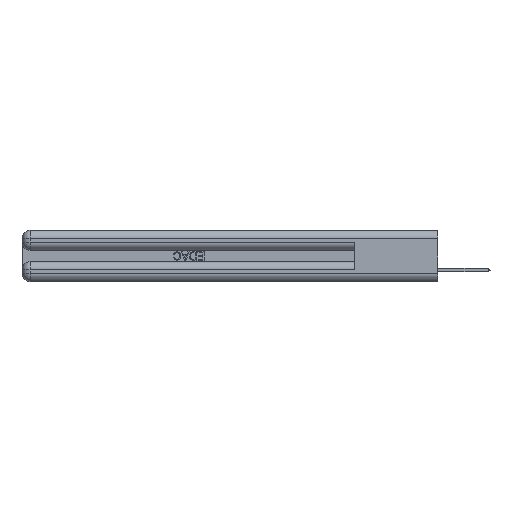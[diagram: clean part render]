
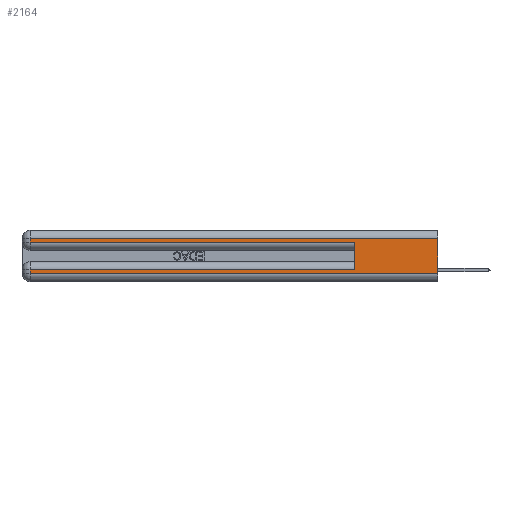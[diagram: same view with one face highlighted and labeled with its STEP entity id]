
A CAD part, left-side view. The second image highlights one B-rep face of the part: STEP entity #2164.
In plain terms, the highlighted planar face has unit normal (-1, 0, 0).
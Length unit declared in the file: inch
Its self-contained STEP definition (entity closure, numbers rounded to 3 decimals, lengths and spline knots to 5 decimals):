
#159 = EDGE_CURVE ( 'NONE', #7602, #18989, #10091, .T. ) ;
#1267 = LINE ( 'NONE', #23984, #44156 ) ;
#2164 = ADVANCED_FACE ( 'NONE', ( #12031 ), #34060, .F. ) ;
#2642 = ORIENTED_EDGE ( 'NONE', *, *, #159, .T. ) ;
#2807 = ORIENTED_EDGE ( 'NONE', *, *, #13919, .F. ) ;
#2818 = EDGE_CURVE ( 'NONE', #22507, #7602, #30417, .T. ) ;
#3405 = ORIENTED_EDGE ( 'NONE', *, *, #26136, .T. ) ;
#4474 = CARTESIAN_POINT ( 'NONE',  ( 0., 0.6, 0.145 ) ) ;
#4896 = AXIS2_PLACEMENT_3D ( 'NONE', #23490, #34382, #41384 ) ;
#6411 = EDGE_CURVE ( 'NONE', #44815, #10000, #44076, .T. ) ;
#6507 = CARTESIAN_POINT ( 'NONE',  ( 0., 0., 0.37 ) ) ;
#6776 = DIRECTION ( 'NONE',  ( 0., 1., 0. ) ) ;
#7141 = CARTESIAN_POINT ( 'NONE',  ( 0., 0.6, 0.085 ) ) ;
#7232 = CARTESIAN_POINT ( 'NONE',  ( 0., 0., 0.06 ) ) ;
#7307 = LINE ( 'NONE', #16290, #10110 ) ;
#7602 = VERTEX_POINT ( 'NONE', #23586 ) ;
#8119 = EDGE_CURVE ( 'NONE', #18989, #27806, #22187, .T. ) ;
#9535 = ORIENTED_EDGE ( 'NONE', *, *, #2818, .T. ) ;
#10000 = VERTEX_POINT ( 'NONE', #22575 ) ;
#10091 = LINE ( 'NONE', #32590, #18378 ) ;
#10110 = VECTOR ( 'NONE', #44787, 39.37008 ) ;
#10791 = DIRECTION ( 'NONE',  ( 0., 0., -1. ) ) ;
#12031 = FACE_OUTER_BOUND ( 'NONE', #30155, .T. ) ;
#12616 = CARTESIAN_POINT ( 'NONE',  ( 0., 0.6, 0.285 ) ) ;
#12782 = VECTOR ( 'NONE', #21292, 39.37008 ) ;
#13919 = EDGE_CURVE ( 'NONE', #22507, #20232, #15907, .T. ) ;
#15163 = CARTESIAN_POINT ( 'NONE',  ( 0., 2.94, 0.06 ) ) ;
#15520 = EDGE_CURVE ( 'NONE', #10000, #19739, #1267, .T. ) ;
#15907 = LINE ( 'NONE', #6507, #18165 ) ;
#16290 = CARTESIAN_POINT ( 'NONE',  ( 0., 0., 0.06 ) ) ;
#16591 = ORIENTED_EDGE ( 'NONE', *, *, #15520, .T. ) ;
#17574 = DIRECTION ( 'NONE',  ( 0., 1., 0. ) ) ;
#18165 = VECTOR ( 'NONE', #10791, 39.37008 ) ;
#18378 = VECTOR ( 'NONE', #40500, 39.37008 ) ;
#18989 = VERTEX_POINT ( 'NONE', #19274 ) ;
#19274 = CARTESIAN_POINT ( 'NONE',  ( 0., 2.94, 0.285 ) ) ;
#19739 = VERTEX_POINT ( 'NONE', #15163 ) ;
#20232 = VERTEX_POINT ( 'NONE', #7232 ) ;
#20900 = EDGE_CURVE ( 'NONE', #44815, #27806, #31871, .T. ) ;
#21292 = DIRECTION ( 'NONE',  ( 0., -1., 0. ) ) ;
#21804 = VECTOR ( 'NONE', #6776, 39.37008 ) ;
#22187 = LINE ( 'NONE', #44348, #12782 ) ;
#22360 = VECTOR ( 'NONE', #33080, 39.37008 ) ;
#22507 = VERTEX_POINT ( 'NONE', #27233 ) ;
#22575 = CARTESIAN_POINT ( 'NONE',  ( 0., 2.94, 0.085 ) ) ;
#23191 = VECTOR ( 'NONE', #17574, 39.37008 ) ;
#23490 = CARTESIAN_POINT ( 'NONE',  ( 0., 0., 0.37 ) ) ;
#23586 = CARTESIAN_POINT ( 'NONE',  ( 0., 2.94, 0.31 ) ) ;
#23871 = ORIENTED_EDGE ( 'NONE', *, *, #6411, .T. ) ;
#23984 = CARTESIAN_POINT ( 'NONE',  ( 0., 2.94, 0.37 ) ) ;
#24438 = CARTESIAN_POINT ( 'NONE',  ( 0., 0., 0.31 ) ) ;
#24493 = ORIENTED_EDGE ( 'NONE', *, *, #20900, .F. ) ;
#26136 = EDGE_CURVE ( 'NONE', #19739, #20232, #7307, .T. ) ;
#27233 = CARTESIAN_POINT ( 'NONE',  ( 0., 0., 0.31 ) ) ;
#27806 = VERTEX_POINT ( 'NONE', #12616 ) ;
#28037 = CARTESIAN_POINT ( 'NONE',  ( 0., 0., 0.085 ) ) ;
#30155 = EDGE_LOOP ( 'NONE', ( #2807, #9535, #2642, #40774, #24493, #23871, #16591, #3405 ) ) ;
#30417 = LINE ( 'NONE', #24438, #23191 ) ;
#31871 = LINE ( 'NONE', #4474, #22360 ) ;
#32590 = CARTESIAN_POINT ( 'NONE',  ( 0., 2.94, 0.37 ) ) ;
#33080 = DIRECTION ( 'NONE',  ( 0., 0., 1. ) ) ;
#34060 = PLANE ( 'NONE',  #4896 ) ;
#34382 = DIRECTION ( 'NONE',  ( 1., 0., 0. ) ) ;
#40500 = DIRECTION ( 'NONE',  ( 0., 0., -1. ) ) ;
#40774 = ORIENTED_EDGE ( 'NONE', *, *, #8119, .T. ) ;
#41384 = DIRECTION ( 'NONE',  ( 0., 0., -1. ) ) ;
#44076 = LINE ( 'NONE', #28037, #21804 ) ;
#44156 = VECTOR ( 'NONE', #45447, 39.37008 ) ;
#44348 = CARTESIAN_POINT ( 'NONE',  ( 0., 0., 0.285 ) ) ;
#44787 = DIRECTION ( 'NONE',  ( 0., -1., 0. ) ) ;
#44815 = VERTEX_POINT ( 'NONE', #7141 ) ;
#45447 = DIRECTION ( 'NONE',  ( 0., 0., -1. ) ) ;
